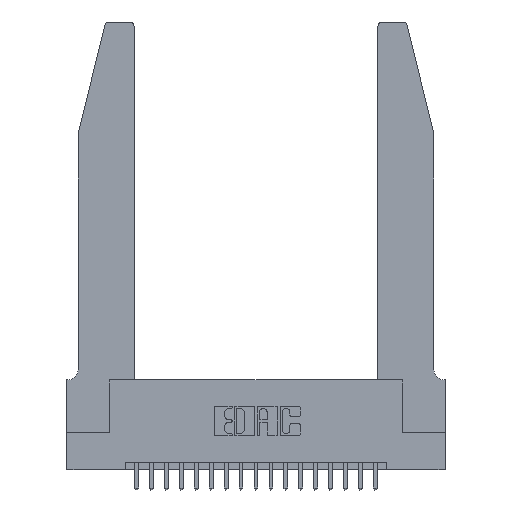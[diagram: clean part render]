
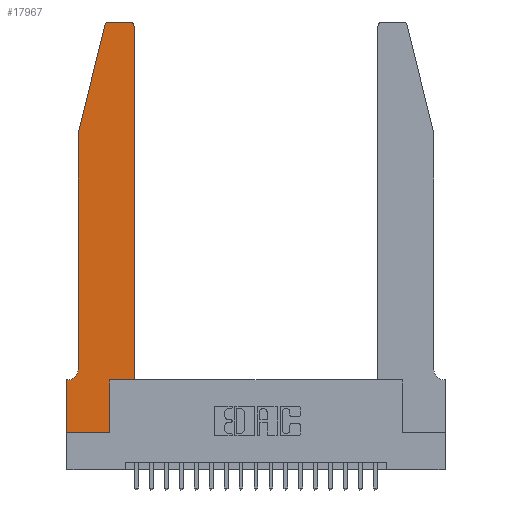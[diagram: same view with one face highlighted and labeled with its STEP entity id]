
A CAD part, top view. The second image highlights one B-rep face of the part: STEP entity #17967.
In plain terms, the highlighted planar face has unit normal (0, 0, 1).
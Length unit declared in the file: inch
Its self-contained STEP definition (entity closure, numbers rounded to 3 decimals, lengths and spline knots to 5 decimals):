
#29 = VERTEX_POINT ( 'NONE', #16968 ) ;
#151 = VECTOR ( 'NONE', #6044, 39.37008 ) ;
#617 = VERTEX_POINT ( 'NONE', #7718 ) ;
#702 = LINE ( 'NONE', #15284, #3522 ) ;
#833 = VERTEX_POINT ( 'NONE', #19701 ) ;
#1257 = LINE ( 'NONE', #19586, #3583 ) ;
#1283 = DIRECTION ( 'NONE',  ( 1., 0., 0. ) ) ;
#1347 = EDGE_LOOP ( 'NONE', ( #4780, #9135, #15741, #13837, #13284, #19482, #17841, #10389, #18030, #7550, #20392, #6594 ) ) ;
#1701 = EDGE_CURVE ( 'NONE', #617, #3912, #1257, .T. ) ;
#1710 = DIRECTION ( 'NONE',  ( 0., 0., 1. ) ) ;
#1851 = CARTESIAN_POINT ( 'NONE',  ( 0.4505, 0.35, 0.37 ) ) ;
#2156 = CARTESIAN_POINT ( 'NONE',  ( 0., 0., 0.37 ) ) ;
#2238 = LINE ( 'NONE', #11431, #14439 ) ;
#2510 = VERTEX_POINT ( 'NONE', #3301 ) ;
#3173 = AXIS2_PLACEMENT_3D ( 'NONE', #4412, #4477, #1283 ) ;
#3301 = CARTESIAN_POINT ( 'NONE',  ( 0.4205, 2.75, 0.37 ) ) ;
#3507 = CARTESIAN_POINT ( 'NONE',  ( 0.4205, 2.72, 0.37 ) ) ;
#3522 = VECTOR ( 'NONE', #13904, 39.37008 ) ;
#3583 = VECTOR ( 'NONE', #13895, 39.37008 ) ;
#3603 = EDGE_CURVE ( 'NONE', #21357, #833, #14678, .T. ) ;
#3912 = VERTEX_POINT ( 'NONE', #12907 ) ;
#4412 = CARTESIAN_POINT ( 'NONE',  ( 0.284, 2.72, 0.37 ) ) ;
#4477 = DIRECTION ( 'NONE',  ( 0., 0., 1. ) ) ;
#4780 = ORIENTED_EDGE ( 'NONE', *, *, #6059, .T. ) ;
#5433 = LINE ( 'NONE', #2156, #16843 ) ;
#5935 = EDGE_CURVE ( 'NONE', #11441, #29, #5433, .T. ) ;
#6044 = DIRECTION ( 'NONE',  ( 0., -1., 0. ) ) ;
#6059 = EDGE_CURVE ( 'NONE', #2510, #14622, #17633, .T. ) ;
#6131 = CARTESIAN_POINT ( 'NONE',  ( 0., 0., 0.37 ) ) ;
#6155 = DIRECTION ( 'NONE',  ( -1., 0., 0. ) ) ;
#6274 = CIRCLE ( 'NONE', #10898, 0.03 ) ;
#6594 = ORIENTED_EDGE ( 'NONE', *, *, #14013, .T. ) ;
#6646 = AXIS2_PLACEMENT_3D ( 'NONE', #13163, #14714, #11508 ) ;
#6941 = DIRECTION ( 'NONE',  ( 0., -1., 0. ) ) ;
#6962 = VERTEX_POINT ( 'NONE', #16055 ) ;
#7550 = ORIENTED_EDGE ( 'NONE', *, *, #11918, .T. ) ;
#7718 = CARTESIAN_POINT ( 'NONE',  ( 0.25487, 2.72718, 0.37 ) ) ;
#8186 = CARTESIAN_POINT ( 'NONE',  ( 0.2865, 0.35, 0.37 ) ) ;
#8246 = DIRECTION ( 'NONE',  ( -1., 0., 0. ) ) ;
#8625 = EDGE_CURVE ( 'NONE', #12728, #11441, #14713, .T. ) ;
#8929 = CARTESIAN_POINT ( 'NONE',  ( 0.2605, 2.75, 0.37 ) ) ;
#8976 = EDGE_CURVE ( 'NONE', #20882, #12728, #2238, .T. ) ;
#9133 = VERTEX_POINT ( 'NONE', #11035 ) ;
#9135 = ORIENTED_EDGE ( 'NONE', *, *, #19458, .T. ) ;
#9438 = EDGE_CURVE ( 'NONE', #3912, #6962, #15964, .T. ) ;
#9503 = CARTESIAN_POINT ( 'NONE',  ( 0.0055, 0.42, 0.37 ) ) ;
#9685 = CARTESIAN_POINT ( 'NONE',  ( 0.284, 2.75, 0.37 ) ) ;
#9698 = LINE ( 'NONE', #8186, #12582 ) ;
#10389 = ORIENTED_EDGE ( 'NONE', *, *, #5935, .T. ) ;
#10552 = DIRECTION ( 'NONE',  ( -1., 0., 0. ) ) ;
#10898 = AXIS2_PLACEMENT_3D ( 'NONE', #3507, #1710, #11650 ) ;
#11035 = CARTESIAN_POINT ( 'NONE',  ( 0.2865, 0.35, 0.37 ) ) ;
#11216 = CARTESIAN_POINT ( 'NONE',  ( 0.4505, 0.35, 0.37 ) ) ;
#11431 = CARTESIAN_POINT ( 'NONE',  ( 0.0755, 0.35, 0.37 ) ) ;
#11441 = VERTEX_POINT ( 'NONE', #6131 ) ;
#11508 = DIRECTION ( 'NONE',  ( 1., 0., 0. ) ) ;
#11650 = DIRECTION ( 'NONE',  ( 1., 0., 0. ) ) ;
#11918 = EDGE_CURVE ( 'NONE', #9133, #21357, #702, .T. ) ;
#12108 = DIRECTION ( 'NONE',  ( 1., 0., 0. ) ) ;
#12582 = VECTOR ( 'NONE', #18324, 39.37008 ) ;
#12599 = VECTOR ( 'NONE', #6941, 39.37008 ) ;
#12728 = VERTEX_POINT ( 'NONE', #20571 ) ;
#12907 = CARTESIAN_POINT ( 'NONE',  ( 0.0755, 2., 0.37 ) ) ;
#13163 = CARTESIAN_POINT ( 'NONE',  ( 0., 0.35, 0.37 ) ) ;
#13284 = ORIENTED_EDGE ( 'NONE', *, *, #13668, .T. ) ;
#13594 = CIRCLE ( 'NONE', #13987, 0.07 ) ;
#13668 = EDGE_CURVE ( 'NONE', #6962, #20882, #13594, .T. ) ;
#13837 = ORIENTED_EDGE ( 'NONE', *, *, #9438, .T. ) ;
#13895 = DIRECTION ( 'NONE',  ( -0.239, -0.971, 0. ) ) ;
#13904 = DIRECTION ( 'NONE',  ( 1., 0., 0. ) ) ;
#13987 = AXIS2_PLACEMENT_3D ( 'NONE', #9503, #16177, #6155 ) ;
#14013 = EDGE_CURVE ( 'NONE', #833, #2510, #6274, .T. ) ;
#14439 = VECTOR ( 'NONE', #8246, 39.37008 ) ;
#14622 = VERTEX_POINT ( 'NONE', #9685 ) ;
#14657 = FACE_OUTER_BOUND ( 'NONE', #1347, .T. ) ;
#14678 = LINE ( 'NONE', #1851, #15208 ) ;
#14713 = LINE ( 'NONE', #16125, #151 ) ;
#14714 = DIRECTION ( 'NONE',  ( 0., 0., 1. ) ) ;
#15208 = VECTOR ( 'NONE', #18993, 39.37008 ) ;
#15284 = CARTESIAN_POINT ( 'NONE',  ( 0.4505, 0.35, 0.37 ) ) ;
#15741 = ORIENTED_EDGE ( 'NONE', *, *, #1701, .T. ) ;
#15829 = VECTOR ( 'NONE', #10552, 39.37008 ) ;
#15964 = LINE ( 'NONE', #20144, #12599 ) ;
#16055 = CARTESIAN_POINT ( 'NONE',  ( 0.0755, 0.42, 0.37 ) ) ;
#16125 = CARTESIAN_POINT ( 'NONE',  ( 0., 0., 0.37 ) ) ;
#16177 = DIRECTION ( 'NONE',  ( 0., 0., -1. ) ) ;
#16264 = CARTESIAN_POINT ( 'NONE',  ( 0.0055, 0.35, 0.37 ) ) ;
#16843 = VECTOR ( 'NONE', #12108, 39.37008 ) ;
#16968 = CARTESIAN_POINT ( 'NONE',  ( 0.2865, 0., 0.37 ) ) ;
#17633 = LINE ( 'NONE', #8929, #15829 ) ;
#17841 = ORIENTED_EDGE ( 'NONE', *, *, #8625, .T. ) ;
#17967 = ADVANCED_FACE ( 'NONE', ( #14657 ), #18174, .T. ) ;
#17974 = EDGE_CURVE ( 'NONE', #29, #9133, #9698, .T. ) ;
#18030 = ORIENTED_EDGE ( 'NONE', *, *, #17974, .T. ) ;
#18174 = PLANE ( 'NONE',  #6646 ) ;
#18324 = DIRECTION ( 'NONE',  ( 0., 1., 0. ) ) ;
#18993 = DIRECTION ( 'NONE',  ( 0., 1., 0. ) ) ;
#19248 = CIRCLE ( 'NONE', #3173, 0.03 ) ;
#19458 = EDGE_CURVE ( 'NONE', #14622, #617, #19248, .T. ) ;
#19482 = ORIENTED_EDGE ( 'NONE', *, *, #8976, .T. ) ;
#19586 = CARTESIAN_POINT ( 'NONE',  ( 0.0755, 2., 0.37 ) ) ;
#19701 = CARTESIAN_POINT ( 'NONE',  ( 0.4505, 2.72, 0.37 ) ) ;
#20144 = CARTESIAN_POINT ( 'NONE',  ( 0.0755, 2., 0.37 ) ) ;
#20392 = ORIENTED_EDGE ( 'NONE', *, *, #3603, .T. ) ;
#20571 = CARTESIAN_POINT ( 'NONE',  ( 0., 0.35, 0.37 ) ) ;
#20882 = VERTEX_POINT ( 'NONE', #16264 ) ;
#21357 = VERTEX_POINT ( 'NONE', #11216 ) ;
